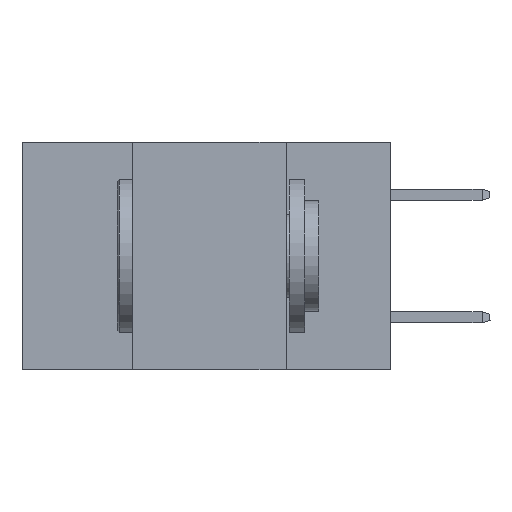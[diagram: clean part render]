
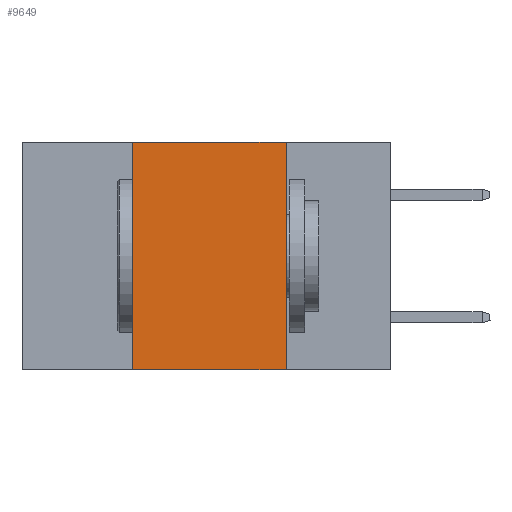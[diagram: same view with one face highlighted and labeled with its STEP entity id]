
A CAD part, left-side view. The second image highlights one B-rep face of the part: STEP entity #9649.
In plain terms, the highlighted planar face has unit normal (-1, 0, 0).
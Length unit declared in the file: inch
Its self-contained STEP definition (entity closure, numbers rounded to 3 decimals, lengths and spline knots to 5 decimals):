
#365 = VERTEX_POINT ( 'NONE', #21931 ) ;
#2767 = CARTESIAN_POINT ( 'NONE',  ( 0., 0.17, 0. ) ) ;
#2886 = LINE ( 'NONE', #5963, #5755 ) ;
#3713 = CARTESIAN_POINT ( 'NONE',  ( 0., 0.42, 0. ) ) ;
#4269 = EDGE_CURVE ( 'NONE', #365, #12578, #13406, .T. ) ;
#4543 = VERTEX_POINT ( 'NONE', #18210 ) ;
#5117 = EDGE_CURVE ( 'NONE', #21319, #365, #20375, .T. ) ;
#5755 = VECTOR ( 'NONE', #19660, 39.37008 ) ;
#5963 = CARTESIAN_POINT ( 'NONE',  ( 0., 0.6, -0.37 ) ) ;
#5987 = VECTOR ( 'NONE', #11328, 39.37008 ) ;
#6432 = AXIS2_PLACEMENT_3D ( 'NONE', #7814, #11445, #15282 ) ;
#6601 = EDGE_CURVE ( 'NONE', #4543, #21319, #23766, .T. ) ;
#7814 = CARTESIAN_POINT ( 'NONE',  ( 0., 0.6, 0. ) ) ;
#8813 = ORIENTED_EDGE ( 'NONE', *, *, #11942, .T. ) ;
#9418 = VECTOR ( 'NONE', #22375, 39.37008 ) ;
#9649 = ADVANCED_FACE ( 'NONE', ( #22095 ), #17514, .F. ) ;
#10307 = VECTOR ( 'NONE', #17429, 39.37008 ) ;
#11328 = DIRECTION ( 'NONE',  ( 0., -1., 0. ) ) ;
#11445 = DIRECTION ( 'NONE',  ( 1., 0., 0. ) ) ;
#11942 = EDGE_CURVE ( 'NONE', #4543, #12578, #2886, .T. ) ;
#12578 = VERTEX_POINT ( 'NONE', #12726 ) ;
#12726 = CARTESIAN_POINT ( 'NONE',  ( 0., 0.17, -0.37 ) ) ;
#13106 = CARTESIAN_POINT ( 'NONE',  ( 0., 0.42, 0. ) ) ;
#13365 = EDGE_LOOP ( 'NONE', ( #18020, #13880, #24747, #8813 ) ) ;
#13406 = LINE ( 'NONE', #2767, #9418 ) ;
#13880 = ORIENTED_EDGE ( 'NONE', *, *, #5117, .F. ) ;
#15282 = DIRECTION ( 'NONE',  ( 0., 0., -1. ) ) ;
#17429 = DIRECTION ( 'NONE',  ( 0., 0., 1. ) ) ;
#17514 = PLANE ( 'NONE',  #6432 ) ;
#18020 = ORIENTED_EDGE ( 'NONE', *, *, #4269, .F. ) ;
#18210 = CARTESIAN_POINT ( 'NONE',  ( 0., 0.42, -0.37 ) ) ;
#19660 = DIRECTION ( 'NONE',  ( 0., -1., 0. ) ) ;
#20375 = LINE ( 'NONE', #24861, #5987 ) ;
#21319 = VERTEX_POINT ( 'NONE', #13106 ) ;
#21931 = CARTESIAN_POINT ( 'NONE',  ( 0., 0.17, 0. ) ) ;
#22095 = FACE_OUTER_BOUND ( 'NONE', #13365, .T. ) ;
#22375 = DIRECTION ( 'NONE',  ( 0., 0., -1. ) ) ;
#23766 = LINE ( 'NONE', #3713, #10307 ) ;
#24747 = ORIENTED_EDGE ( 'NONE', *, *, #6601, .F. ) ;
#24861 = CARTESIAN_POINT ( 'NONE',  ( 0., 0.6, 0. ) ) ;
